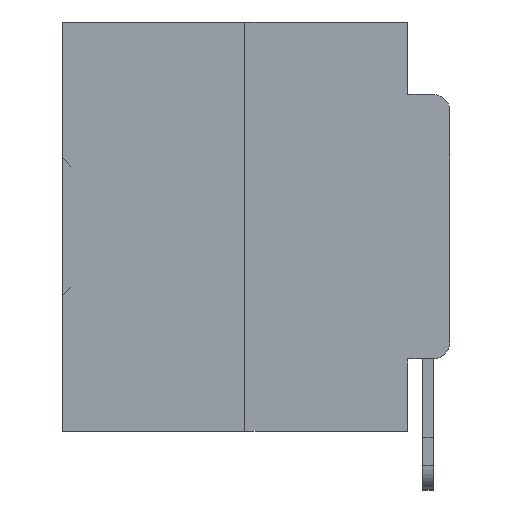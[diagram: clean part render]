
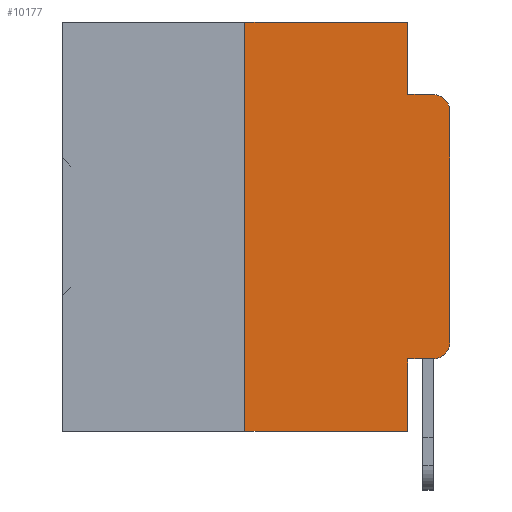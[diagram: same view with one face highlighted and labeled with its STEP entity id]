
A CAD part, left-side view. The second image highlights one B-rep face of the part: STEP entity #10177.
In plain terms, the highlighted planar face has unit normal (-1, 0, 0).
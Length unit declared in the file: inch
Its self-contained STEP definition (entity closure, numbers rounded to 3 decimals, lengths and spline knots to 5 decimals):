
#251 = LINE ( 'NONE', #28084, #1188 ) ;
#889 = VECTOR ( 'NONE', #31292, 39.37008 ) ;
#1188 = VECTOR ( 'NONE', #10023, 39.37008 ) ;
#3073 = CARTESIAN_POINT ( 'NONE',  ( 0., 0.25, 0. ) ) ;
#3273 = LINE ( 'NONE', #35488, #10362 ) ;
#3598 = FACE_OUTER_BOUND ( 'NONE', #29586, .T. ) ;
#3798 = CARTESIAN_POINT ( 'NONE',  ( 0., 0.02, -0.1085 ) ) ;
#4290 = CARTESIAN_POINT ( 'NONE',  ( 0., 0.051, 0. ) ) ;
#5365 = CARTESIAN_POINT ( 'NONE',  ( 0., 0.02, -0.3915 ) ) ;
#5764 = LINE ( 'NONE', #33801, #20887 ) ;
#6828 = DIRECTION ( 'NONE',  ( 0., 0., -1. ) ) ;
#7010 = VERTEX_POINT ( 'NONE', #37230 ) ;
#7360 = ORIENTED_EDGE ( 'NONE', *, *, #11058, .F. ) ;
#7540 = VERTEX_POINT ( 'NONE', #4290 ) ;
#7908 = VERTEX_POINT ( 'NONE', #3073 ) ;
#8027 = CARTESIAN_POINT ( 'NONE',  ( 0., 0., -0.3915 ) ) ;
#8406 = DIRECTION ( 'NONE',  ( 0., 0., -1. ) ) ;
#9157 = ORIENTED_EDGE ( 'NONE', *, *, #21703, .F. ) ;
#9322 = ORIENTED_EDGE ( 'NONE', *, *, #38377, .F. ) ;
#10023 = DIRECTION ( 'NONE',  ( 0., 0., -1. ) ) ;
#10104 = EDGE_CURVE ( 'NONE', #22056, #11227, #15425, .T. ) ;
#10177 = ADVANCED_FACE ( 'NONE', ( #3598 ), #31206, .F. ) ;
#10273 = DIRECTION ( 'NONE',  ( 1., 0., 0. ) ) ;
#10362 = VECTOR ( 'NONE', #38450, 39.37008 ) ;
#10500 = EDGE_CURVE ( 'NONE', #21497, #10780, #21257, .T. ) ;
#10780 = VERTEX_POINT ( 'NONE', #22359 ) ;
#11039 = ORIENTED_EDGE ( 'NONE', *, *, #17119, .F. ) ;
#11058 = EDGE_CURVE ( 'NONE', #13142, #10780, #3273, .T. ) ;
#11227 = VERTEX_POINT ( 'NONE', #18380 ) ;
#11573 = DIRECTION ( 'NONE',  ( 0., -1., 0. ) ) ;
#11623 = CARTESIAN_POINT ( 'NONE',  ( 0., 0., -0.1085 ) ) ;
#11940 = CARTESIAN_POINT ( 'NONE',  ( 0., 0., 0. ) ) ;
#12811 = DIRECTION ( 'NONE',  ( 0., 0., 1. ) ) ;
#13025 = VERTEX_POINT ( 'NONE', #8027 ) ;
#13142 = VERTEX_POINT ( 'NONE', #14626 ) ;
#13174 = ORIENTED_EDGE ( 'NONE', *, *, #22671, .T. ) ;
#14325 = CARTESIAN_POINT ( 'NONE',  ( 0., 0.051, -0.0885 ) ) ;
#14626 = CARTESIAN_POINT ( 'NONE',  ( 0., 0.051, -0.4115 ) ) ;
#15394 = AXIS2_PLACEMENT_3D ( 'NONE', #3798, #24920, #6828 ) ;
#15425 = CIRCLE ( 'NONE', #15394, 0.02 ) ;
#15864 = CARTESIAN_POINT ( 'NONE',  ( 0., 0.051, -0.0885 ) ) ;
#16297 = CARTESIAN_POINT ( 'NONE',  ( 0., 0.473, 0. ) ) ;
#16336 = AXIS2_PLACEMENT_3D ( 'NONE', #5365, #26470, #8406 ) ;
#17119 = EDGE_CURVE ( 'NONE', #21497, #7908, #5764, .T. ) ;
#17137 = LINE ( 'NONE', #15864, #30345 ) ;
#18380 = CARTESIAN_POINT ( 'NONE',  ( 0., 0.02, -0.0885 ) ) ;
#19636 = VECTOR ( 'NONE', #11573, 39.37008 ) ;
#19929 = VERTEX_POINT ( 'NONE', #14325 ) ;
#20298 = ORIENTED_EDGE ( 'NONE', *, *, #10500, .T. ) ;
#20887 = VECTOR ( 'NONE', #12811, 39.37008 ) ;
#21257 = LINE ( 'NONE', #24096, #36161 ) ;
#21471 = EDGE_CURVE ( 'NONE', #13025, #22056, #29893, .T. ) ;
#21497 = VERTEX_POINT ( 'NONE', #32959 ) ;
#21703 = EDGE_CURVE ( 'NONE', #19929, #11227, #17137, .T. ) ;
#22056 = VERTEX_POINT ( 'NONE', #11623 ) ;
#22359 = CARTESIAN_POINT ( 'NONE',  ( 0., 0.051, -0.5 ) ) ;
#22671 = EDGE_CURVE ( 'NONE', #7010, #13025, #32135, .T. ) ;
#24096 = CARTESIAN_POINT ( 'NONE',  ( 0., 0.473, -0.5 ) ) ;
#24920 = DIRECTION ( 'NONE',  ( -1., 0., 0. ) ) ;
#25007 = LINE ( 'NONE', #16297, #889 ) ;
#26470 = DIRECTION ( 'NONE',  ( -1., 0., 0. ) ) ;
#27688 = LINE ( 'NONE', #32610, #19636 ) ;
#28084 = CARTESIAN_POINT ( 'NONE',  ( 0., 0.051, 0. ) ) ;
#28433 = ORIENTED_EDGE ( 'NONE', *, *, #21471, .T. ) ;
#29586 = EDGE_LOOP ( 'NONE', ( #28433, #35988, #9157, #9322, #33980, #11039, #20298, #7360, #36882, #13174 ) ) ;
#29893 = LINE ( 'NONE', #11940, #37703 ) ;
#30151 = DIRECTION ( 'NONE',  ( 0., -1., 0. ) ) ;
#30345 = VECTOR ( 'NONE', #30999, 39.37008 ) ;
#30999 = DIRECTION ( 'NONE',  ( 0., -1., 0. ) ) ;
#31206 = PLANE ( 'NONE',  #35430 ) ;
#31292 = DIRECTION ( 'NONE',  ( 0., -1., 0. ) ) ;
#31330 = DIRECTION ( 'NONE',  ( 0., 0., -1. ) ) ;
#32135 = CIRCLE ( 'NONE', #16336, 0.02 ) ;
#32610 = CARTESIAN_POINT ( 'NONE',  ( 0., 0.051, -0.4115 ) ) ;
#32959 = CARTESIAN_POINT ( 'NONE',  ( 0., 0.25, -0.5 ) ) ;
#33801 = CARTESIAN_POINT ( 'NONE',  ( 0., 0.25, 0. ) ) ;
#33962 = EDGE_CURVE ( 'NONE', #13142, #7010, #27688, .T. ) ;
#33980 = ORIENTED_EDGE ( 'NONE', *, *, #36403, .F. ) ;
#35430 = AXIS2_PLACEMENT_3D ( 'NONE', #37089, #10273, #31330 ) ;
#35488 = CARTESIAN_POINT ( 'NONE',  ( 0., 0.051, 0. ) ) ;
#35871 = DIRECTION ( 'NONE',  ( 0., 0., 1. ) ) ;
#35988 = ORIENTED_EDGE ( 'NONE', *, *, #10104, .T. ) ;
#36161 = VECTOR ( 'NONE', #30151, 39.37008 ) ;
#36403 = EDGE_CURVE ( 'NONE', #7908, #7540, #25007, .T. ) ;
#36882 = ORIENTED_EDGE ( 'NONE', *, *, #33962, .T. ) ;
#37089 = CARTESIAN_POINT ( 'NONE',  ( 0., 0.473, 0. ) ) ;
#37230 = CARTESIAN_POINT ( 'NONE',  ( 0., 0.02, -0.4115 ) ) ;
#37703 = VECTOR ( 'NONE', #35871, 39.37008 ) ;
#38377 = EDGE_CURVE ( 'NONE', #7540, #19929, #251, .T. ) ;
#38450 = DIRECTION ( 'NONE',  ( 0., 0., -1. ) ) ;
